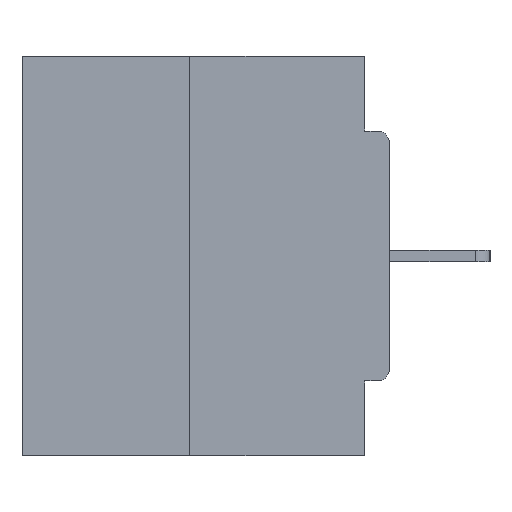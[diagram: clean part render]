
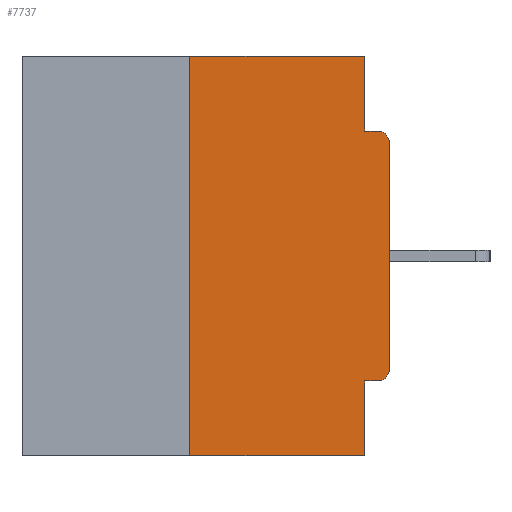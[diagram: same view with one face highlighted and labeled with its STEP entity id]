
A CAD part, left-side view. The second image highlights one B-rep face of the part: STEP entity #7737.
In plain terms, the highlighted planar face has unit normal (-1, 0, 0).
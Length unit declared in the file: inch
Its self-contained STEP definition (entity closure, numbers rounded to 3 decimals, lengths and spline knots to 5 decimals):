
#1497 = EDGE_CURVE ( 'NONE', #23257, #22565, #27627, .T. ) ;
#1627 = VECTOR ( 'NONE', #18683, 39.37008 ) ;
#1830 = VECTOR ( 'NONE', #20257, 39.37008 ) ;
#2011 = CARTESIAN_POINT ( 'NONE',  ( 0., 0.015, -0.0935 ) ) ;
#2253 = EDGE_CURVE ( 'NONE', #13412, #17312, #28224, .T. ) ;
#2360 = ORIENTED_EDGE ( 'NONE', *, *, #15907, .F. ) ;
#2708 = VECTOR ( 'NONE', #21164, 39.37008 ) ;
#3703 = EDGE_CURVE ( 'NONE', #29368, #9649, #26169, .T. ) ;
#3859 = DIRECTION ( 'NONE',  ( 1., 0., 0. ) ) ;
#4331 = EDGE_CURVE ( 'NONE', #22565, #17364, #19555, .T. ) ;
#4833 = DIRECTION ( 'NONE',  ( 0., 0., 1. ) ) ;
#4861 = DIRECTION ( 'NONE',  ( 0., 1., 0. ) ) ;
#5187 = CARTESIAN_POINT ( 'NONE',  ( 0., 0.25, -0.5 ) ) ;
#5329 = CARTESIAN_POINT ( 'NONE',  ( 0., 0.25, 0. ) ) ;
#5828 = AXIS2_PLACEMENT_3D ( 'NONE', #20119, #29581, #8314 ) ;
#6721 = EDGE_CURVE ( 'NONE', #30512, #9259, #11990, .T. ) ;
#6772 = VECTOR ( 'NONE', #24695, 39.37008 ) ;
#6829 = CARTESIAN_POINT ( 'NONE',  ( 0., 0.015, -0.4065 ) ) ;
#7186 = ORIENTED_EDGE ( 'NONE', *, *, #13786, .F. ) ;
#7202 = CARTESIAN_POINT ( 'NONE',  ( 0., 0., -0.4065 ) ) ;
#7424 = ORIENTED_EDGE ( 'NONE', *, *, #20990, .F. ) ;
#7472 = CARTESIAN_POINT ( 'NONE',  ( 0., 0.031, 0. ) ) ;
#7516 = CARTESIAN_POINT ( 'NONE',  ( 0., 0.031, -0.5 ) ) ;
#7692 = EDGE_LOOP ( 'NONE', ( #10674, #2360, #30013, #29753, #7424, #24822, #27547, #12919, #7186, #15962 ) ) ;
#7737 = ADVANCED_FACE ( 'NONE', ( #8698 ), #18025, .F. ) ;
#8314 = DIRECTION ( 'NONE',  ( 0., 0., -1. ) ) ;
#8698 = FACE_OUTER_BOUND ( 'NONE', #7692, .T. ) ;
#8822 = CARTESIAN_POINT ( 'NONE',  ( 0., 0.031, -0.5 ) ) ;
#9259 = VERTEX_POINT ( 'NONE', #8822 ) ;
#9519 = LINE ( 'NONE', #30621, #2708 ) ;
#9649 = VERTEX_POINT ( 'NONE', #26505 ) ;
#9748 = DIRECTION ( 'NONE',  ( 0., 0., -1. ) ) ;
#9914 = EDGE_CURVE ( 'NONE', #9649, #13412, #9519, .T. ) ;
#9933 = DIRECTION ( 'NONE',  ( 0., 0., -1. ) ) ;
#9981 = CARTESIAN_POINT ( 'NONE',  ( 0., 0.25, 0. ) ) ;
#10011 = LINE ( 'NONE', #7202, #29230 ) ;
#10674 = ORIENTED_EDGE ( 'NONE', *, *, #1497, .F. ) ;
#10787 = CARTESIAN_POINT ( 'NONE',  ( 0., 0., -0.0935 ) ) ;
#11031 = CARTESIAN_POINT ( 'NONE',  ( 0., 0.46, 0. ) ) ;
#11066 = EDGE_CURVE ( 'NONE', #26405, #9259, #17159, .T. ) ;
#11661 = CARTESIAN_POINT ( 'NONE',  ( 0., 0.031, -0.0935 ) ) ;
#11990 = LINE ( 'NONE', #30622, #1627 ) ;
#12558 = CARTESIAN_POINT ( 'NONE',  ( 0., 0.031, 0. ) ) ;
#12620 = VECTOR ( 'NONE', #4833, 39.37008 ) ;
#12919 = ORIENTED_EDGE ( 'NONE', *, *, #2253, .T. ) ;
#13412 = VERTEX_POINT ( 'NONE', #30363 ) ;
#13786 = EDGE_CURVE ( 'NONE', #17364, #17312, #24903, .T. ) ;
#15365 = AXIS2_PLACEMENT_3D ( 'NONE', #21691, #29130, #9748 ) ;
#15907 = EDGE_CURVE ( 'NONE', #30512, #23257, #24086, .T. ) ;
#15962 = ORIENTED_EDGE ( 'NONE', *, *, #4331, .F. ) ;
#16791 = VECTOR ( 'NONE', #9933, 39.37008 ) ;
#17159 = LINE ( 'NONE', #7516, #28551 ) ;
#17312 = VERTEX_POINT ( 'NONE', #2011 ) ;
#17364 = VERTEX_POINT ( 'NONE', #11661 ) ;
#17720 = CARTESIAN_POINT ( 'NONE',  ( 0., 0.46, 0. ) ) ;
#17871 = DIRECTION ( 'NONE',  ( 0., 0., -1. ) ) ;
#18025 = PLANE ( 'NONE',  #21934 ) ;
#18233 = CARTESIAN_POINT ( 'NONE',  ( 0., 0.031, -0.4065 ) ) ;
#18683 = DIRECTION ( 'NONE',  ( 0., -1., 0. ) ) ;
#19178 = DIRECTION ( 'NONE',  ( 0., 0., -1. ) ) ;
#19555 = LINE ( 'NONE', #12558, #16791 ) ;
#20119 = CARTESIAN_POINT ( 'NONE',  ( 0., 0.015, -0.3915 ) ) ;
#20257 = DIRECTION ( 'NONE',  ( 0., -1., 0. ) ) ;
#20990 = EDGE_CURVE ( 'NONE', #29368, #26405, #10011, .T. ) ;
#21164 = DIRECTION ( 'NONE',  ( 0., 0., 1. ) ) ;
#21691 = CARTESIAN_POINT ( 'NONE',  ( 0., 0.015, -0.1085 ) ) ;
#21934 = AXIS2_PLACEMENT_3D ( 'NONE', #17720, #3859, #17871 ) ;
#22565 = VERTEX_POINT ( 'NONE', #7472 ) ;
#23257 = VERTEX_POINT ( 'NONE', #5329 ) ;
#24086 = LINE ( 'NONE', #9981, #12620 ) ;
#24695 = DIRECTION ( 'NONE',  ( 0., -1., 0. ) ) ;
#24822 = ORIENTED_EDGE ( 'NONE', *, *, #3703, .T. ) ;
#24903 = LINE ( 'NONE', #10787, #1830 ) ;
#26169 = CIRCLE ( 'NONE', #5828, 0.015 ) ;
#26405 = VERTEX_POINT ( 'NONE', #18233 ) ;
#26505 = CARTESIAN_POINT ( 'NONE',  ( 0., 0., -0.3915 ) ) ;
#27547 = ORIENTED_EDGE ( 'NONE', *, *, #9914, .T. ) ;
#27627 = LINE ( 'NONE', #11031, #6772 ) ;
#28224 = CIRCLE ( 'NONE', #15365, 0.015 ) ;
#28551 = VECTOR ( 'NONE', #19178, 39.37008 ) ;
#29130 = DIRECTION ( 'NONE',  ( -1., 0., 0. ) ) ;
#29230 = VECTOR ( 'NONE', #4861, 39.37008 ) ;
#29368 = VERTEX_POINT ( 'NONE', #6829 ) ;
#29581 = DIRECTION ( 'NONE',  ( -1., 0., 0. ) ) ;
#29753 = ORIENTED_EDGE ( 'NONE', *, *, #11066, .F. ) ;
#30013 = ORIENTED_EDGE ( 'NONE', *, *, #6721, .T. ) ;
#30363 = CARTESIAN_POINT ( 'NONE',  ( 0., 0., -0.1085 ) ) ;
#30512 = VERTEX_POINT ( 'NONE', #5187 ) ;
#30621 = CARTESIAN_POINT ( 'NONE',  ( 0., 0., 0. ) ) ;
#30622 = CARTESIAN_POINT ( 'NONE',  ( 0., 0.46, -0.5 ) ) ;
